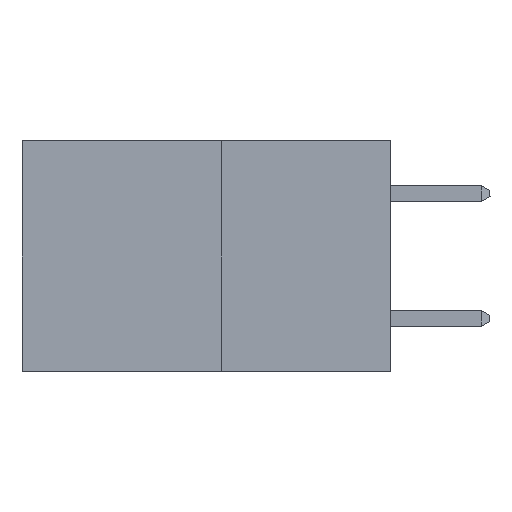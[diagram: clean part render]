
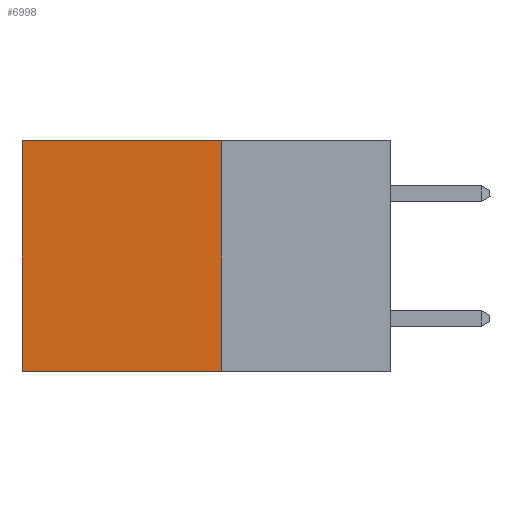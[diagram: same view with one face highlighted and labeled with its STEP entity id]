
A CAD part, left-side view. The second image highlights one B-rep face of the part: STEP entity #6998.
In plain terms, the highlighted planar face has unit normal (-1, 0, 0).
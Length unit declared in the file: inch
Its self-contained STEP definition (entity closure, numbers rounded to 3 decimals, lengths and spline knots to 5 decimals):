
#45 = ORIENTED_EDGE ( 'NONE', *, *, #14173, .T. ) ;
#984 = VECTOR ( 'NONE', #14235, 39.37008 ) ;
#1019 = CARTESIAN_POINT ( 'NONE',  ( 0.277, 0.59, -0.37 ) ) ;
#1739 = CARTESIAN_POINT ( 'NONE',  ( 0.277, 0.27, -0.37 ) ) ;
#1823 = DIRECTION ( 'NONE',  ( 0., 0., -1. ) ) ;
#1947 = EDGE_LOOP ( 'NONE', ( #45, #19770, #7935, #19268 ) ) ;
#1948 = VERTEX_POINT ( 'NONE', #2213 ) ;
#2213 = CARTESIAN_POINT ( 'NONE',  ( 0.277, 0.27, -0.37 ) ) ;
#2552 = AXIS2_PLACEMENT_3D ( 'NONE', #1739, #13996, #1823 ) ;
#4449 = DIRECTION ( 'NONE',  ( 0., 1., 0. ) ) ;
#4555 = DIRECTION ( 'NONE',  ( 0., 0., -1. ) ) ;
#6188 = FACE_OUTER_BOUND ( 'NONE', #1947, .T. ) ;
#6998 = ADVANCED_FACE ( 'NONE', ( #6188 ), #11989, .F. ) ;
#7935 = ORIENTED_EDGE ( 'NONE', *, *, #14267, .F. ) ;
#8064 = CARTESIAN_POINT ( 'NONE',  ( 0.277, 0.59, 0. ) ) ;
#8227 = LINE ( 'NONE', #16664, #12997 ) ;
#8988 = CARTESIAN_POINT ( 'NONE',  ( 0.277, 0.27, -0.37 ) ) ;
#9998 = VECTOR ( 'NONE', #15060, 39.37008 ) ;
#10622 = LINE ( 'NONE', #8988, #9998 ) ;
#11989 = PLANE ( 'NONE',  #2552 ) ;
#12997 = VECTOR ( 'NONE', #4555, 39.37008 ) ;
#13996 = DIRECTION ( 'NONE',  ( 1., 0., 0. ) ) ;
#14173 = EDGE_CURVE ( 'NONE', #17602, #25610, #8227, .T. ) ;
#14235 = DIRECTION ( 'NONE',  ( 0., 0., -1. ) ) ;
#14267 = EDGE_CURVE ( 'NONE', #18570, #1948, #22319, .T. ) ;
#14741 = EDGE_CURVE ( 'NONE', #18570, #17602, #20345, .T. ) ;
#15060 = DIRECTION ( 'NONE',  ( 0., 1., 0. ) ) ;
#16664 = CARTESIAN_POINT ( 'NONE',  ( 0.277, 0.59, -0.37 ) ) ;
#17198 = EDGE_CURVE ( 'NONE', #1948, #25610, #10622, .T. ) ;
#17602 = VERTEX_POINT ( 'NONE', #8064 ) ;
#18570 = VERTEX_POINT ( 'NONE', #24832 ) ;
#19268 = ORIENTED_EDGE ( 'NONE', *, *, #14741, .T. ) ;
#19770 = ORIENTED_EDGE ( 'NONE', *, *, #17198, .F. ) ;
#20345 = LINE ( 'NONE', #20481, #25653 ) ;
#20481 = CARTESIAN_POINT ( 'NONE',  ( 0.277, 0.27, 0. ) ) ;
#22319 = LINE ( 'NONE', #24058, #984 ) ;
#24058 = CARTESIAN_POINT ( 'NONE',  ( 0.277, 0.27, -0.37 ) ) ;
#24832 = CARTESIAN_POINT ( 'NONE',  ( 0.277, 0.27, 0. ) ) ;
#25610 = VERTEX_POINT ( 'NONE', #1019 ) ;
#25653 = VECTOR ( 'NONE', #4449, 39.37008 ) ;
